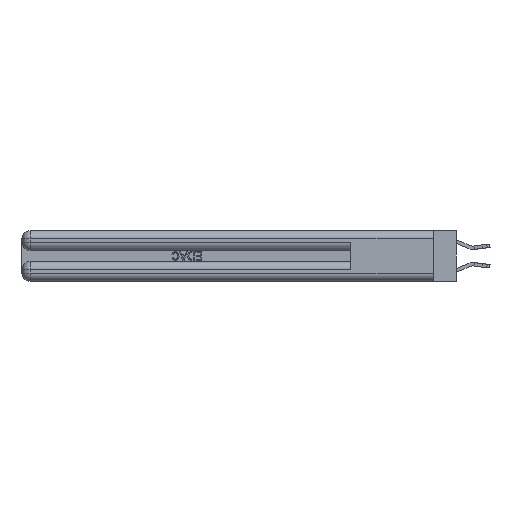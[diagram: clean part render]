
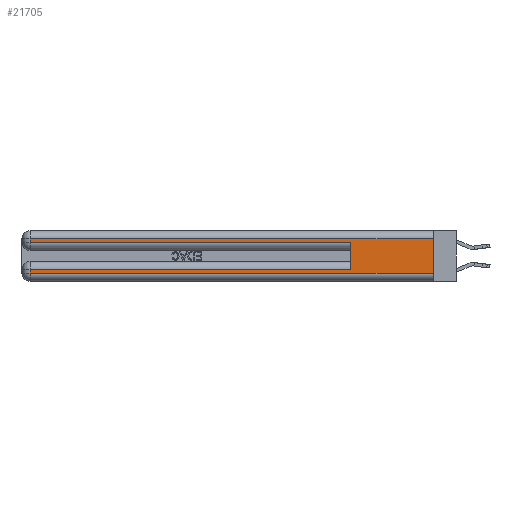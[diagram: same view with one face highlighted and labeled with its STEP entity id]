
A CAD part, left-side view. The second image highlights one B-rep face of the part: STEP entity #21705.
In plain terms, the highlighted planar face has unit normal (-1, 0, 0).
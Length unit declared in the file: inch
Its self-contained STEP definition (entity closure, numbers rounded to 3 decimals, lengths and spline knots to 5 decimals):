
#709 = VECTOR ( 'NONE', #12649, 39.37008 ) ;
#1003 = VERTEX_POINT ( 'NONE', #15449 ) ;
#1023 = LINE ( 'NONE', #7547, #25420 ) ;
#1869 = ORIENTED_EDGE ( 'NONE', *, *, #8263, .F. ) ;
#2394 = EDGE_CURVE ( 'NONE', #1003, #13411, #7864, .T. ) ;
#2804 = DIRECTION ( 'NONE',  ( 0., 1., 0. ) ) ;
#2916 = VECTOR ( 'NONE', #24134, 39.37008 ) ;
#3184 = CARTESIAN_POINT ( 'NONE',  ( 0., 2.94, 0.37 ) ) ;
#3592 = ORIENTED_EDGE ( 'NONE', *, *, #25283, .T. ) ;
#3602 = LINE ( 'NONE', #14291, #709 ) ;
#3671 = VERTEX_POINT ( 'NONE', #28745 ) ;
#3930 = LINE ( 'NONE', #15081, #2916 ) ;
#5046 = ORIENTED_EDGE ( 'NONE', *, *, #16735, .T. ) ;
#5699 = LINE ( 'NONE', #3184, #28693 ) ;
#5860 = LINE ( 'NONE', #10626, #15713 ) ;
#6012 = DIRECTION ( 'NONE',  ( 0., 0., 1. ) ) ;
#6013 = ORIENTED_EDGE ( 'NONE', *, *, #14245, .T. ) ;
#6088 = VERTEX_POINT ( 'NONE', #16145 ) ;
#7233 = FACE_OUTER_BOUND ( 'NONE', #23568, .T. ) ;
#7311 = CARTESIAN_POINT ( 'NONE',  ( 0., 0., 0.285 ) ) ;
#7547 = CARTESIAN_POINT ( 'NONE',  ( 0., 0., 0.31 ) ) ;
#7864 = LINE ( 'NONE', #16932, #27679 ) ;
#8263 = EDGE_CURVE ( 'NONE', #24683, #12136, #3602, .T. ) ;
#8929 = VERTEX_POINT ( 'NONE', #15586 ) ;
#10626 = CARTESIAN_POINT ( 'NONE',  ( 0., 0.6, 0.145 ) ) ;
#12136 = VERTEX_POINT ( 'NONE', #19159 ) ;
#12649 = DIRECTION ( 'NONE',  ( 0., 0., -1. ) ) ;
#12980 = CARTESIAN_POINT ( 'NONE',  ( 0., 0., 0.085 ) ) ;
#13271 = LINE ( 'NONE', #12980, #24340 ) ;
#13332 = EDGE_CURVE ( 'NONE', #13411, #18221, #27696, .T. ) ;
#13411 = VERTEX_POINT ( 'NONE', #22404 ) ;
#13891 = ORIENTED_EDGE ( 'NONE', *, *, #2394, .T. ) ;
#14245 = EDGE_CURVE ( 'NONE', #8929, #6088, #13271, .T. ) ;
#14291 = CARTESIAN_POINT ( 'NONE',  ( 0., 0., 0.37 ) ) ;
#14354 = DIRECTION ( 'NONE',  ( 0., 0., -1. ) ) ;
#15081 = CARTESIAN_POINT ( 'NONE',  ( 0., 0., 0.06 ) ) ;
#15449 = CARTESIAN_POINT ( 'NONE',  ( 0., 2.94, 0.31 ) ) ;
#15586 = CARTESIAN_POINT ( 'NONE',  ( 0., 0.6, 0.085 ) ) ;
#15713 = VECTOR ( 'NONE', #6012, 39.37008 ) ;
#16145 = CARTESIAN_POINT ( 'NONE',  ( 0., 2.94, 0.085 ) ) ;
#16382 = DIRECTION ( 'NONE',  ( 0., -1., 0. ) ) ;
#16618 = ORIENTED_EDGE ( 'NONE', *, *, #13332, .T. ) ;
#16735 = EDGE_CURVE ( 'NONE', #6088, #3671, #5699, .T. ) ;
#16932 = CARTESIAN_POINT ( 'NONE',  ( 0., 2.94, 0.37 ) ) ;
#18221 = VERTEX_POINT ( 'NONE', #18682 ) ;
#18682 = CARTESIAN_POINT ( 'NONE',  ( 0., 0.6, 0.285 ) ) ;
#18827 = CARTESIAN_POINT ( 'NONE',  ( 0., 0., 0.37 ) ) ;
#19159 = CARTESIAN_POINT ( 'NONE',  ( 0., 0., 0.06 ) ) ;
#19404 = ORIENTED_EDGE ( 'NONE', *, *, #25990, .T. ) ;
#20733 = VECTOR ( 'NONE', #16382, 39.37008 ) ;
#20913 = PLANE ( 'NONE',  #27232 ) ;
#21705 = ADVANCED_FACE ( 'NONE', ( #7233 ), #20913, .F. ) ;
#22404 = CARTESIAN_POINT ( 'NONE',  ( 0., 2.94, 0.285 ) ) ;
#23568 = EDGE_LOOP ( 'NONE', ( #1869, #3592, #13891, #16618, #28823, #6013, #5046, #19404 ) ) ;
#24134 = DIRECTION ( 'NONE',  ( 0., -1., 0. ) ) ;
#24340 = VECTOR ( 'NONE', #26675, 39.37008 ) ;
#24683 = VERTEX_POINT ( 'NONE', #25140 ) ;
#25140 = CARTESIAN_POINT ( 'NONE',  ( 0., 0., 0.31 ) ) ;
#25283 = EDGE_CURVE ( 'NONE', #24683, #1003, #1023, .T. ) ;
#25420 = VECTOR ( 'NONE', #2804, 39.37008 ) ;
#25930 = DIRECTION ( 'NONE',  ( 0., 0., -1. ) ) ;
#25974 = EDGE_CURVE ( 'NONE', #8929, #18221, #5860, .T. ) ;
#25990 = EDGE_CURVE ( 'NONE', #3671, #12136, #3930, .T. ) ;
#26004 = DIRECTION ( 'NONE',  ( 0., 0., -1. ) ) ;
#26675 = DIRECTION ( 'NONE',  ( 0., 1., 0. ) ) ;
#27232 = AXIS2_PLACEMENT_3D ( 'NONE', #18827, #27764, #14354 ) ;
#27679 = VECTOR ( 'NONE', #26004, 39.37008 ) ;
#27696 = LINE ( 'NONE', #7311, #20733 ) ;
#27764 = DIRECTION ( 'NONE',  ( 1., 0., 0. ) ) ;
#28693 = VECTOR ( 'NONE', #25930, 39.37008 ) ;
#28745 = CARTESIAN_POINT ( 'NONE',  ( 0., 2.94, 0.06 ) ) ;
#28823 = ORIENTED_EDGE ( 'NONE', *, *, #25974, .F. ) ;
